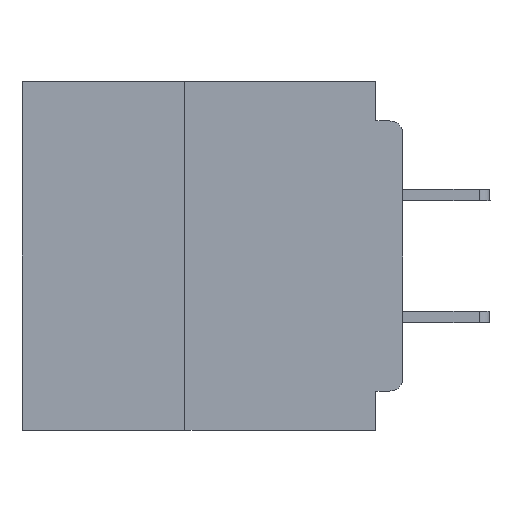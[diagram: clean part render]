
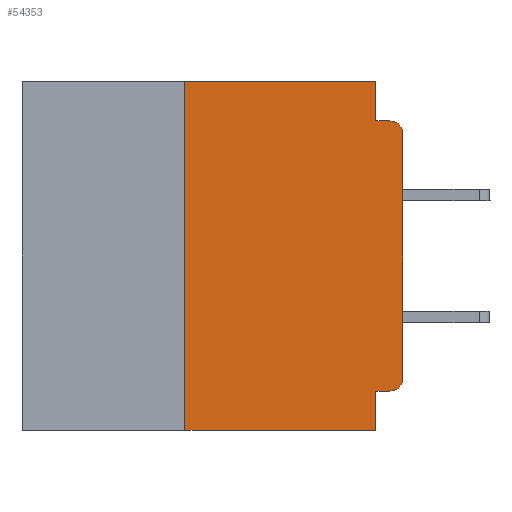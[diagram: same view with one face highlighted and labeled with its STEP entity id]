
A CAD part, left-side view. The second image highlights one B-rep face of the part: STEP entity #54353.
In plain terms, the highlighted planar face has unit normal (-1, 0, 0).
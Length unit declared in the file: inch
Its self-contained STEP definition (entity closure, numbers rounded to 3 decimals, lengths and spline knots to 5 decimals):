
#58 = CARTESIAN_POINT ( 'NONE',  ( 0., 0., -0.06 ) ) ;
#718 = CARTESIAN_POINT ( 'NONE',  ( 0., 0.437, -0.4 ) ) ;
#1132 = CARTESIAN_POINT ( 'NONE',  ( 0., 0.25, -0.4 ) ) ;
#4143 = VECTOR ( 'NONE', #36828, 39.37008 ) ;
#5341 = LINE ( 'NONE', #718, #47503 ) ;
#5354 = VECTOR ( 'NONE', #17636, 39.37008 ) ;
#5909 = VERTEX_POINT ( 'NONE', #18741 ) ;
#6202 = ORIENTED_EDGE ( 'NONE', *, *, #59370, .F. ) ;
#6533 = ORIENTED_EDGE ( 'NONE', *, *, #28529, .F. ) ;
#7366 = ORIENTED_EDGE ( 'NONE', *, *, #30595, .F. ) ;
#7798 = FACE_OUTER_BOUND ( 'NONE', #12787, .T. ) ;
#7850 = CARTESIAN_POINT ( 'NONE',  ( 0., 0.437, 0. ) ) ;
#8009 = VERTEX_POINT ( 'NONE', #65279 ) ;
#8204 = VERTEX_POINT ( 'NONE', #56625 ) ;
#8726 = EDGE_CURVE ( 'NONE', #22959, #49348, #21124, .T. ) ;
#8783 = DIRECTION ( 'NONE',  ( 0., 0., -1. ) ) ;
#9716 = CARTESIAN_POINT ( 'NONE',  ( 0., 0.031, -0.4 ) ) ;
#10676 = CARTESIAN_POINT ( 'NONE',  ( 0., 0.25, -0.4 ) ) ;
#10857 = CARTESIAN_POINT ( 'NONE',  ( 0., 0.015, -0.34 ) ) ;
#12288 = CARTESIAN_POINT ( 'NONE',  ( 0., 0.015, -0.355 ) ) ;
#12787 = EDGE_LOOP ( 'NONE', ( #45035, #32984, #6533, #7366, #54802, #6202, #29342, #53768, #35286, #59755 ) ) ;
#12999 = DIRECTION ( 'NONE',  ( 0., 0., 1. ) ) ;
#13025 = EDGE_CURVE ( 'NONE', #32014, #23761, #5341, .T. ) ;
#15009 = LINE ( 'NONE', #59419, #52258 ) ;
#16059 = DIRECTION ( 'NONE',  ( 0., 0., -1. ) ) ;
#17296 = AXIS2_PLACEMENT_3D ( 'NONE', #10857, #46356, #16059 ) ;
#17636 = DIRECTION ( 'NONE',  ( 0., 0., -1. ) ) ;
#18221 = PLANE ( 'NONE',  #65252 ) ;
#18741 = CARTESIAN_POINT ( 'NONE',  ( 0., 0.25, 0. ) ) ;
#21124 = CIRCLE ( 'NONE', #17296, 0.015 ) ;
#21886 = LINE ( 'NONE', #27974, #47178 ) ;
#22043 = VERTEX_POINT ( 'NONE', #58 ) ;
#22226 = LINE ( 'NONE', #37791, #5354 ) ;
#22581 = VECTOR ( 'NONE', #12999, 39.37008 ) ;
#22959 = VERTEX_POINT ( 'NONE', #12288 ) ;
#23290 = DIRECTION ( 'NONE',  ( 1., 0., 0. ) ) ;
#23761 = VERTEX_POINT ( 'NONE', #9716 ) ;
#23856 = DIRECTION ( 'NONE',  ( -1., 0., 0. ) ) ;
#25731 = DIRECTION ( 'NONE',  ( 0., -1., 0. ) ) ;
#27974 = CARTESIAN_POINT ( 'NONE',  ( 0., 0., -0.355 ) ) ;
#28529 = EDGE_CURVE ( 'NONE', #8009, #8204, #32769, .T. ) ;
#29342 = ORIENTED_EDGE ( 'NONE', *, *, #13025, .T. ) ;
#30595 = EDGE_CURVE ( 'NONE', #38088, #8009, #15009, .T. ) ;
#31122 = DIRECTION ( 'NONE',  ( 0., -1., 0. ) ) ;
#32014 = VERTEX_POINT ( 'NONE', #10676 ) ;
#32769 = LINE ( 'NONE', #50950, #58102 ) ;
#32984 = ORIENTED_EDGE ( 'NONE', *, *, #64945, .T. ) ;
#33089 = DIRECTION ( 'NONE',  ( 0., 1., 0. ) ) ;
#34046 = DIRECTION ( 'NONE',  ( 0., -1., 0. ) ) ;
#35286 = ORIENTED_EDGE ( 'NONE', *, *, #50560, .F. ) ;
#36283 = VECTOR ( 'NONE', #34046, 39.37008 ) ;
#36828 = DIRECTION ( 'NONE',  ( 0., 0., 1. ) ) ;
#37791 = CARTESIAN_POINT ( 'NONE',  ( 0., 0.031, -0.4 ) ) ;
#38088 = VERTEX_POINT ( 'NONE', #44129 ) ;
#39397 = EDGE_CURVE ( 'NONE', #48500, #23761, #22226, .T. ) ;
#39828 = AXIS2_PLACEMENT_3D ( 'NONE', #54209, #23856, #59302 ) ;
#40827 = EDGE_CURVE ( 'NONE', #5909, #38088, #49700, .T. ) ;
#44129 = CARTESIAN_POINT ( 'NONE',  ( 0., 0.031, 0. ) ) ;
#44743 = LINE ( 'NONE', #1132, #4143 ) ;
#45035 = ORIENTED_EDGE ( 'NONE', *, *, #51255, .T. ) ;
#45041 = CARTESIAN_POINT ( 'NONE',  ( 0., 0.031, -0.355 ) ) ;
#45783 = CIRCLE ( 'NONE', #39828, 0.015 ) ;
#46356 = DIRECTION ( 'NONE',  ( -1., 0., 0. ) ) ;
#47178 = VECTOR ( 'NONE', #33089, 39.37008 ) ;
#47503 = VECTOR ( 'NONE', #31122, 39.37008 ) ;
#47890 = LINE ( 'NONE', #48677, #22581 ) ;
#48500 = VERTEX_POINT ( 'NONE', #45041 ) ;
#48677 = CARTESIAN_POINT ( 'NONE',  ( 0., 0., 0. ) ) ;
#49348 = VERTEX_POINT ( 'NONE', #61822 ) ;
#49700 = LINE ( 'NONE', #59285, #36283 ) ;
#50560 = EDGE_CURVE ( 'NONE', #22959, #48500, #21886, .T. ) ;
#50950 = CARTESIAN_POINT ( 'NONE',  ( 0., 0., -0.045 ) ) ;
#51255 = EDGE_CURVE ( 'NONE', #49348, #22043, #47890, .T. ) ;
#52258 = VECTOR ( 'NONE', #8783, 39.37008 ) ;
#53768 = ORIENTED_EDGE ( 'NONE', *, *, #39397, .F. ) ;
#54209 = CARTESIAN_POINT ( 'NONE',  ( 0., 0.015, -0.06 ) ) ;
#54353 = ADVANCED_FACE ( 'NONE', ( #7798 ), #18221, .F. ) ;
#54802 = ORIENTED_EDGE ( 'NONE', *, *, #40827, .F. ) ;
#56625 = CARTESIAN_POINT ( 'NONE',  ( 0., 0.015, -0.045 ) ) ;
#58102 = VECTOR ( 'NONE', #25731, 39.37008 ) ;
#58728 = DIRECTION ( 'NONE',  ( 0., 0., -1. ) ) ;
#59285 = CARTESIAN_POINT ( 'NONE',  ( 0., 0.437, 0. ) ) ;
#59302 = DIRECTION ( 'NONE',  ( 0., 0., -1. ) ) ;
#59370 = EDGE_CURVE ( 'NONE', #32014, #5909, #44743, .T. ) ;
#59419 = CARTESIAN_POINT ( 'NONE',  ( 0., 0.031, 0. ) ) ;
#59755 = ORIENTED_EDGE ( 'NONE', *, *, #8726, .T. ) ;
#61822 = CARTESIAN_POINT ( 'NONE',  ( 0., 0., -0.34 ) ) ;
#64945 = EDGE_CURVE ( 'NONE', #22043, #8204, #45783, .T. ) ;
#65252 = AXIS2_PLACEMENT_3D ( 'NONE', #7850, #23290, #58728 ) ;
#65279 = CARTESIAN_POINT ( 'NONE',  ( 0., 0.031, -0.045 ) ) ;
